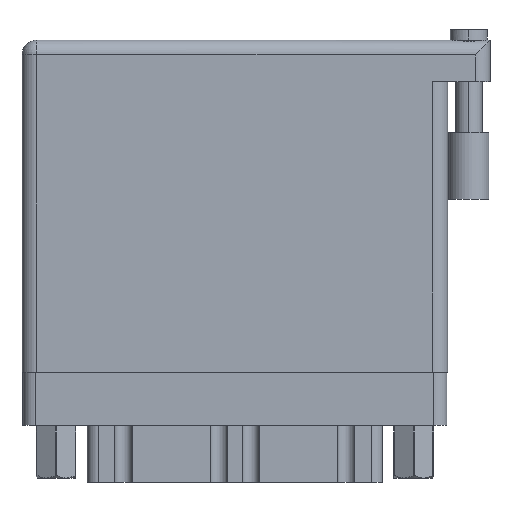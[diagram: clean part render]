
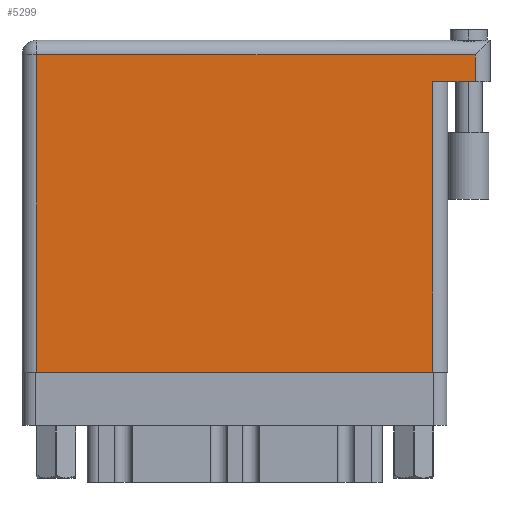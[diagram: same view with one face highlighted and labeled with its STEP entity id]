
A CAD part, front view. The second image highlights one B-rep face of the part: STEP entity #5299.
In plain terms, the highlighted face is planar.
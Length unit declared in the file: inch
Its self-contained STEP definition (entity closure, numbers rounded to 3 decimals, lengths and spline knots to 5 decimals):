
#2252 = EDGE_CURVE ( 'NONE', #19800, #28935, #19340, .T. ) ;
#2891 = DIRECTION ( 'NONE',  ( 0., 1., 0. ) ) ;
#3063 = ORIENTED_EDGE ( 'NONE', *, *, #17040, .T. ) ;
#4911 = VECTOR ( 'NONE', #15584, 39.37008 ) ;
#5202 = LINE ( 'NONE', #11361, #10683 ) ;
#5299 = ADVANCED_FACE ( 'NONE', ( #25201 ), #31986, .F. ) ;
#5757 = CARTESIAN_POINT ( 'NONE',  ( 1.938, 0., 0. ) ) ;
#6765 = CARTESIAN_POINT ( 'NONE',  ( 0.07, 0., 0. ) ) ;
#7128 = CARTESIAN_POINT ( 'NONE',  ( 2.138, 1.496, 0. ) ) ;
#8607 = DIRECTION ( 'NONE',  ( 0., 1., 0. ) ) ;
#10683 = VECTOR ( 'NONE', #31948, 39.37008 ) ;
#10855 = VERTEX_POINT ( 'NONE', #25938 ) ;
#11361 = CARTESIAN_POINT ( 'NONE',  ( 0., 0., 0. ) ) ;
#12246 = VECTOR ( 'NONE', #2891, 39.37008 ) ;
#12263 = DIRECTION ( 'NONE',  ( 0., 0., -1. ) ) ;
#12478 = LINE ( 'NONE', #22124, #28309 ) ;
#14685 = EDGE_CURVE ( 'NONE', #19800, #24872, #34267, .T. ) ;
#15584 = DIRECTION ( 'NONE',  ( -1., 0., 0. ) ) ;
#15850 = CARTESIAN_POINT ( 'NONE',  ( 2.138, 1.566, 0. ) ) ;
#16541 = ORIENTED_EDGE ( 'NONE', *, *, #17450, .T. ) ;
#17040 = EDGE_CURVE ( 'NONE', #36098, #24872, #43211, .T. ) ;
#17450 = EDGE_CURVE ( 'NONE', #10855, #30696, #12478, .T. ) ;
#17955 = VECTOR ( 'NONE', #23975, 39.37008 ) ;
#18353 = ORIENTED_EDGE ( 'NONE', *, *, #30904, .T. ) ;
#19229 = CARTESIAN_POINT ( 'NONE',  ( 2.138, 1.369, 0. ) ) ;
#19340 = LINE ( 'NONE', #15850, #43297 ) ;
#19800 = VERTEX_POINT ( 'NONE', #19229 ) ;
#19944 = CARTESIAN_POINT ( 'NONE',  ( 0., 1.496, 0. ) ) ;
#22124 = CARTESIAN_POINT ( 'NONE',  ( 0.07, 0., 0. ) ) ;
#23321 = CARTESIAN_POINT ( 'NONE',  ( 2.208, 1.369, 0. ) ) ;
#23975 = DIRECTION ( 'NONE',  ( -1., 0., 0. ) ) ;
#24872 = VERTEX_POINT ( 'NONE', #35296 ) ;
#25027 = ORIENTED_EDGE ( 'NONE', *, *, #34270, .T. ) ;
#25201 = FACE_OUTER_BOUND ( 'NONE', #27035, .T. ) ;
#25938 = CARTESIAN_POINT ( 'NONE',  ( 0.07, 1.496, 0. ) ) ;
#26050 = DIRECTION ( 'NONE',  ( -1., 0., 0. ) ) ;
#27035 = EDGE_LOOP ( 'NONE', ( #18353, #3063, #33443, #39051, #25027, #16541 ) ) ;
#28309 = VECTOR ( 'NONE', #39202, 39.37008 ) ;
#28610 = AXIS2_PLACEMENT_3D ( 'NONE', #28694, #12263, #26050 ) ;
#28694 = CARTESIAN_POINT ( 'NONE',  ( 0., 1.566, 0. ) ) ;
#28935 = VERTEX_POINT ( 'NONE', #7128 ) ;
#30696 = VERTEX_POINT ( 'NONE', #6765 ) ;
#30904 = EDGE_CURVE ( 'NONE', #30696, #36098, #5202, .T. ) ;
#31948 = DIRECTION ( 'NONE',  ( 1., 0., 0. ) ) ;
#31986 = PLANE ( 'NONE',  #28610 ) ;
#33443 = ORIENTED_EDGE ( 'NONE', *, *, #14685, .F. ) ;
#34267 = LINE ( 'NONE', #23321, #17955 ) ;
#34270 = EDGE_CURVE ( 'NONE', #28935, #10855, #36599, .T. ) ;
#35296 = CARTESIAN_POINT ( 'NONE',  ( 1.938, 1.369, 0. ) ) ;
#36098 = VERTEX_POINT ( 'NONE', #5757 ) ;
#36599 = LINE ( 'NONE', #19944, #4911 ) ;
#39051 = ORIENTED_EDGE ( 'NONE', *, *, #2252, .T. ) ;
#39202 = DIRECTION ( 'NONE',  ( 0., -1., 0. ) ) ;
#42983 = CARTESIAN_POINT ( 'NONE',  ( 1.938, 1.369, 0. ) ) ;
#43211 = LINE ( 'NONE', #42983, #12246 ) ;
#43297 = VECTOR ( 'NONE', #8607, 39.37008 ) ;
